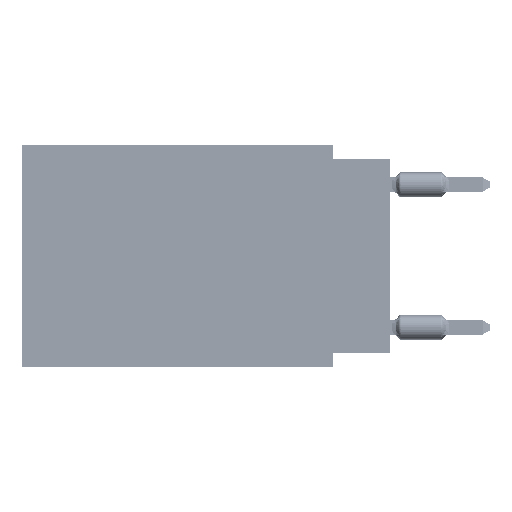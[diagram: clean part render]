
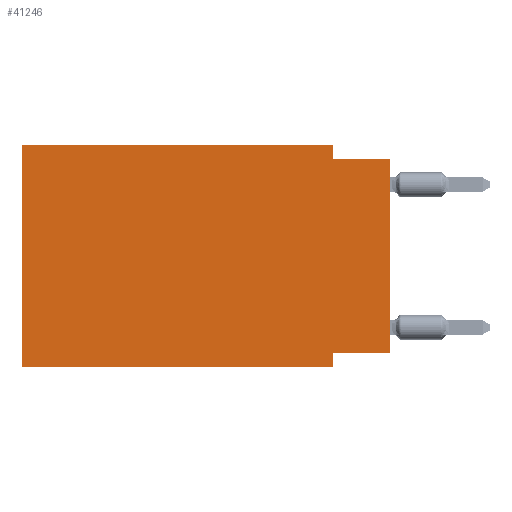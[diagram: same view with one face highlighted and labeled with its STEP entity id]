
A CAD part, left-side view. The second image highlights one B-rep face of the part: STEP entity #41246.
In plain terms, the highlighted planar face has unit normal (-1, 0, 0).
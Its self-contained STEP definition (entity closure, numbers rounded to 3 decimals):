
#1567 = VERTEX_POINT ( 'NONE', #41213 ) ;
#2006 = DIRECTION ( 'NONE',  ( 0., 1., 0. ) ) ;
#4037 = VECTOR ( 'NONE', #35025, 1000. ) ;
#4094 = CARTESIAN_POINT ( 'NONE',  ( 0., 16.383, -9.906 ) ) ;
#4481 = LINE ( 'NONE', #9471, #30487 ) ;
#5109 = CARTESIAN_POINT ( 'NONE',  ( 0., 16.383, 0. ) ) ;
#5198 = ORIENTED_EDGE ( 'NONE', *, *, #47884, .F. ) ;
#6136 = CARTESIAN_POINT ( 'NONE',  ( 0., 0., -9.271 ) ) ;
#8023 = VERTEX_POINT ( 'NONE', #22028 ) ;
#9471 = CARTESIAN_POINT ( 'NONE',  ( 0., 0., -0.635 ) ) ;
#10503 = DIRECTION ( 'NONE',  ( 0., 0., 1. ) ) ;
#10906 = VERTEX_POINT ( 'NONE', #31771 ) ;
#10918 = EDGE_CURVE ( 'NONE', #1567, #78290, #80076, .T. ) ;
#15179 = LINE ( 'NONE', #40397, #4037 ) ;
#15400 = EDGE_CURVE ( 'NONE', #16371, #57089, #33460, .T. ) ;
#16277 = LINE ( 'NONE', #80269, #69795 ) ;
#16371 = VERTEX_POINT ( 'NONE', #6136 ) ;
#16711 = FACE_OUTER_BOUND ( 'NONE', #75822, .T. ) ;
#17125 = DIRECTION ( 'NONE',  ( 1., 0., 0. ) ) ;
#17409 = CARTESIAN_POINT ( 'NONE',  ( 0., 2.54, 0. ) ) ;
#17447 = VECTOR ( 'NONE', #27856, 1000. ) ;
#17826 = CARTESIAN_POINT ( 'NONE',  ( 0., 2.54, -9.906 ) ) ;
#18310 = CARTESIAN_POINT ( 'NONE',  ( 0., 2.54, -9.906 ) ) ;
#22028 = CARTESIAN_POINT ( 'NONE',  ( 0., 0., -0.635 ) ) ;
#27856 = DIRECTION ( 'NONE',  ( 0., -1., 0. ) ) ;
#30487 = VECTOR ( 'NONE', #60277, 1000. ) ;
#31771 = CARTESIAN_POINT ( 'NONE',  ( 0., 2.54, -0.635 ) ) ;
#32236 = ORIENTED_EDGE ( 'NONE', *, *, #15400, .F. ) ;
#33460 = LINE ( 'NONE', #39653, #42002 ) ;
#35025 = DIRECTION ( 'NONE',  ( 0., 0., 1. ) ) ;
#36142 = EDGE_CURVE ( 'NONE', #43805, #1567, #16277, .T. ) ;
#36168 = DIRECTION ( 'NONE',  ( 0., 0., -1. ) ) ;
#37429 = ORIENTED_EDGE ( 'NONE', *, *, #67348, .T. ) ;
#38924 = ORIENTED_EDGE ( 'NONE', *, *, #46855, .F. ) ;
#39116 = LINE ( 'NONE', #71284, #58391 ) ;
#39653 = CARTESIAN_POINT ( 'NONE',  ( 0., 0., -9.271 ) ) ;
#40397 = CARTESIAN_POINT ( 'NONE',  ( 0., 0., 0. ) ) ;
#41213 = CARTESIAN_POINT ( 'NONE',  ( 0., 16.383, 0. ) ) ;
#41246 = ADVANCED_FACE ( 'NONE', ( #16711 ), #67101, .F. ) ;
#42002 = VECTOR ( 'NONE', #2006, 1000. ) ;
#42510 = VECTOR ( 'NONE', #61300, 1000. ) ;
#43805 = VERTEX_POINT ( 'NONE', #4094 ) ;
#46154 = VERTEX_POINT ( 'NONE', #17826 ) ;
#46855 = EDGE_CURVE ( 'NONE', #10906, #8023, #4481, .T. ) ;
#47884 = EDGE_CURVE ( 'NONE', #57089, #46154, #69098, .T. ) ;
#50345 = DIRECTION ( 'NONE',  ( 0., -1., 0. ) ) ;
#51044 = AXIS2_PLACEMENT_3D ( 'NONE', #5109, #17125, #36168 ) ;
#52652 = CARTESIAN_POINT ( 'NONE',  ( 0., 16.383, -9.906 ) ) ;
#56858 = CARTESIAN_POINT ( 'NONE',  ( 0., 2.54, -9.271 ) ) ;
#57089 = VERTEX_POINT ( 'NONE', #56858 ) ;
#57342 = ORIENTED_EDGE ( 'NONE', *, *, #10918, .F. ) ;
#58391 = VECTOR ( 'NONE', #64296, 1000. ) ;
#60277 = DIRECTION ( 'NONE',  ( 0., -1., 0. ) ) ;
#61300 = DIRECTION ( 'NONE',  ( 0., 0., -1. ) ) ;
#64087 = ORIENTED_EDGE ( 'NONE', *, *, #36142, .F. ) ;
#64296 = DIRECTION ( 'NONE',  ( 0., 0., -1. ) ) ;
#64316 = ORIENTED_EDGE ( 'NONE', *, *, #75343, .F. ) ;
#67101 = PLANE ( 'NONE',  #51044 ) ;
#67348 = EDGE_CURVE ( 'NONE', #43805, #46154, #78602, .T. ) ;
#68076 = CARTESIAN_POINT ( 'NONE',  ( 0., 16.383, 0. ) ) ;
#69098 = LINE ( 'NONE', #18310, #42510 ) ;
#69795 = VECTOR ( 'NONE', #10503, 1000. ) ;
#71284 = CARTESIAN_POINT ( 'NONE',  ( 0., 2.54, 0. ) ) ;
#72619 = EDGE_CURVE ( 'NONE', #16371, #8023, #15179, .T. ) ;
#75343 = EDGE_CURVE ( 'NONE', #78290, #10906, #39116, .T. ) ;
#75822 = EDGE_LOOP ( 'NONE', ( #75946, #38924, #64316, #57342, #64087, #37429, #5198, #32236 ) ) ;
#75946 = ORIENTED_EDGE ( 'NONE', *, *, #72619, .T. ) ;
#78290 = VERTEX_POINT ( 'NONE', #17409 ) ;
#78602 = LINE ( 'NONE', #52652, #17447 ) ;
#80076 = LINE ( 'NONE', #68076, #81544 ) ;
#80269 = CARTESIAN_POINT ( 'NONE',  ( 0., 16.383, 0. ) ) ;
#81544 = VECTOR ( 'NONE', #50345, 1000. ) ;
